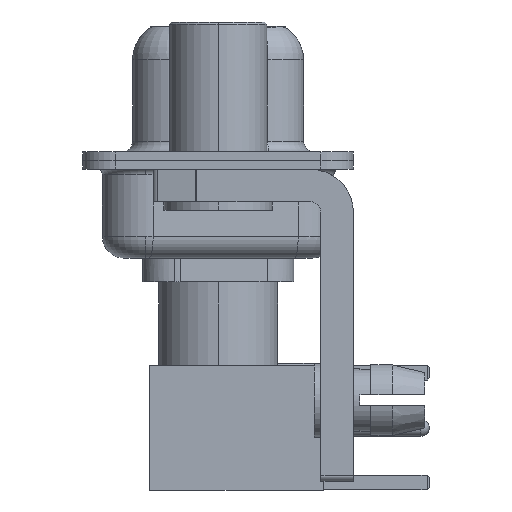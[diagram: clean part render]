
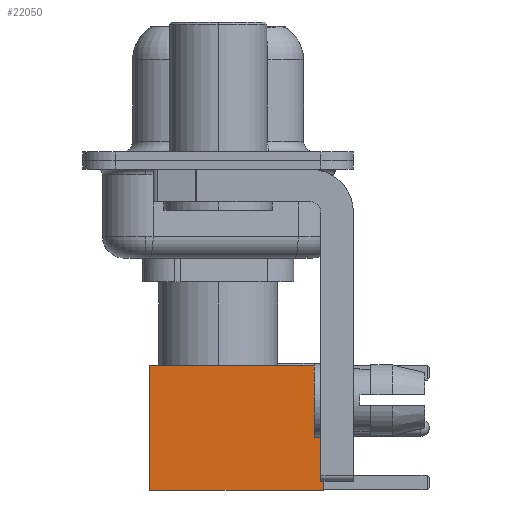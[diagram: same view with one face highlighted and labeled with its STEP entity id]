
A CAD part, left-side view. The second image highlights one B-rep face of the part: STEP entity #22050.
In plain terms, the highlighted face is planar.
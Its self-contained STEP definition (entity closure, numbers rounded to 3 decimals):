
#328 = DIRECTION ( 'NONE',  ( -1., 0., 0. ) ) ;
#960 = LINE ( 'NONE', #8233, #1026 ) ;
#1026 = VECTOR ( 'NONE', #21085, 1000. ) ;
#1368 = DIRECTION ( 'NONE',  ( 0., 0., 1. ) ) ;
#2345 = VERTEX_POINT ( 'NONE', #2764 ) ;
#2764 = CARTESIAN_POINT ( 'NONE',  ( 2.875, 2.875, 8. ) ) ;
#3329 = FACE_OUTER_BOUND ( 'NONE', #4018, .T. ) ;
#4018 = EDGE_LOOP ( 'NONE', ( #4704, #5720, #15028, #5346 ) ) ;
#4526 = CARTESIAN_POINT ( 'NONE',  ( 2.875, 2.875, 0. ) ) ;
#4704 = ORIENTED_EDGE ( 'NONE', *, *, #8261, .T. ) ;
#5300 = EDGE_CURVE ( 'NONE', #2345, #6083, #20696, .T. ) ;
#5318 = PLANE ( 'NONE',  #22712 ) ;
#5346 = ORIENTED_EDGE ( 'NONE', *, *, #5300, .F. ) ;
#5720 = ORIENTED_EDGE ( 'NONE', *, *, #13900, .T. ) ;
#6083 = VERTEX_POINT ( 'NONE', #6939 ) ;
#6939 = CARTESIAN_POINT ( 'NONE',  ( -2.875, 2.875, 8. ) ) ;
#8233 = CARTESIAN_POINT ( 'NONE',  ( -2.875, 2.875, 0. ) ) ;
#8261 = EDGE_CURVE ( 'NONE', #2345, #24191, #20973, .T. ) ;
#9368 = DIRECTION ( 'NONE',  ( -1., 0., 0. ) ) ;
#9496 = VECTOR ( 'NONE', #11099, 1000. ) ;
#11099 = DIRECTION ( 'NONE',  ( 0., 0., -1. ) ) ;
#11423 = CARTESIAN_POINT ( 'NONE',  ( 0., 2.875, 8. ) ) ;
#11475 = CARTESIAN_POINT ( 'NONE',  ( 0., 2.875, 0. ) ) ;
#12153 = VECTOR ( 'NONE', #328, 1000. ) ;
#12594 = CARTESIAN_POINT ( 'NONE',  ( -2.875, 2.875, 0. ) ) ;
#13017 = VECTOR ( 'NONE', #9368, 1000. ) ;
#13792 = VERTEX_POINT ( 'NONE', #12594 ) ;
#13900 = EDGE_CURVE ( 'NONE', #24191, #13792, #15165, .T. ) ;
#15028 = ORIENTED_EDGE ( 'NONE', *, *, #21274, .F. ) ;
#15165 = LINE ( 'NONE', #11475, #13017 ) ;
#20124 = DIRECTION ( 'NONE',  ( 0., 1., 0. ) ) ;
#20696 = LINE ( 'NONE', #11423, #12153 ) ;
#20973 = LINE ( 'NONE', #24354, #9496 ) ;
#21085 = DIRECTION ( 'NONE',  ( 0., 0., -1. ) ) ;
#21274 = EDGE_CURVE ( 'NONE', #6083, #13792, #960, .T. ) ;
#22050 = ADVANCED_FACE ( 'NONE', ( #3329 ), #5318, .T. ) ;
#22598 = CARTESIAN_POINT ( 'NONE',  ( 2.875, 2.875, 0. ) ) ;
#22712 = AXIS2_PLACEMENT_3D ( 'NONE', #22598, #20124, #1368 ) ;
#24191 = VERTEX_POINT ( 'NONE', #4526 ) ;
#24354 = CARTESIAN_POINT ( 'NONE',  ( 2.875, 2.875, 0. ) ) ;
